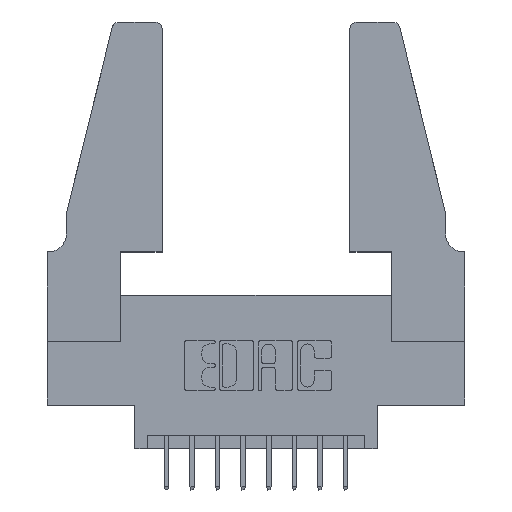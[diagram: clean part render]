
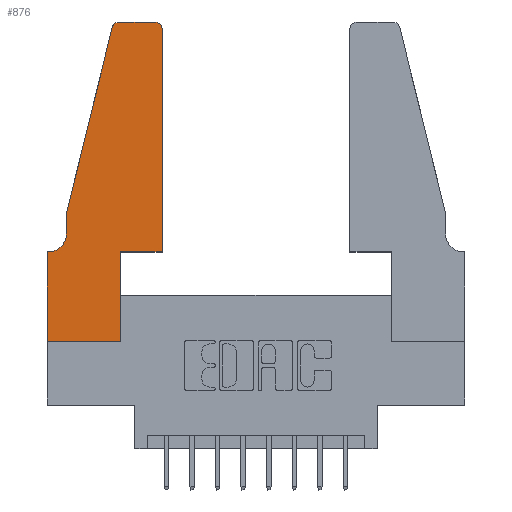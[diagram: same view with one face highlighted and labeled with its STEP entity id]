
A CAD part, top view. The second image highlights one B-rep face of the part: STEP entity #876.
In plain terms, the highlighted planar face has unit normal (0, 0, 1).
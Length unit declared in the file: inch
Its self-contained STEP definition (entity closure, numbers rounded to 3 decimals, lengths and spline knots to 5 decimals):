
#2 = EDGE_CURVE ( 'NONE', #5639, #6989, #9946, .T. ) ;
#331 = VERTEX_POINT ( 'NONE', #1885 ) ;
#429 = EDGE_CURVE ( 'NONE', #331, #4525, #10278, .T. ) ;
#537 = LINE ( 'NONE', #7313, #11053 ) ;
#578 = EDGE_CURVE ( 'NONE', #9862, #8758, #537, .T. ) ;
#680 = ORIENTED_EDGE ( 'NONE', *, *, #429, .T. ) ;
#696 = EDGE_CURVE ( 'NONE', #8758, #331, #12492, .T. ) ;
#757 = DIRECTION ( 'NONE',  ( 0., 1., 0. ) ) ;
#809 = VERTEX_POINT ( 'NONE', #13026 ) ;
#876 = ADVANCED_FACE ( 'NONE', ( #4827 ), #5006, .T. ) ;
#889 = CARTESIAN_POINT ( 'NONE',  ( 0., 0.35, 0.37 ) ) ;
#1090 = DIRECTION ( 'NONE',  ( 1., 0., 0. ) ) ;
#1103 = DIRECTION ( 'NONE',  ( 0., 0., 1. ) ) ;
#1106 = ORIENTED_EDGE ( 'NONE', *, *, #2, .T. ) ;
#1365 = DIRECTION ( 'NONE',  ( 1., 0., 0. ) ) ;
#1399 = VECTOR ( 'NONE', #11381, 39.37008 ) ;
#1441 = VECTOR ( 'NONE', #6751, 39.37008 ) ;
#1780 = CARTESIAN_POINT ( 'NONE',  ( 0.4505, 1.22, 0.37 ) ) ;
#1885 = CARTESIAN_POINT ( 'NONE',  ( 0.0755, 0.42, 0.37 ) ) ;
#1956 = VERTEX_POINT ( 'NONE', #6237 ) ;
#1975 = AXIS2_PLACEMENT_3D ( 'NONE', #5099, #12222, #6137 ) ;
#2273 = EDGE_CURVE ( 'NONE', #11721, #809, #9568, .T. ) ;
#2358 = VECTOR ( 'NONE', #8477, 39.37008 ) ;
#2512 = DIRECTION ( 'NONE',  ( -1., 0., 0. ) ) ;
#3281 = DIRECTION ( 'NONE',  ( -0.239, -0.971, 0. ) ) ;
#3434 = VECTOR ( 'NONE', #1090, 39.37008 ) ;
#3533 = DIRECTION ( 'NONE',  ( 0., 0., 1. ) ) ;
#3571 = ORIENTED_EDGE ( 'NONE', *, *, #10720, .T. ) ;
#3953 = VECTOR ( 'NONE', #2512, 39.37008 ) ;
#4116 = CARTESIAN_POINT ( 'NONE',  ( 0.2865, 0.35, 0.37 ) ) ;
#4489 = CARTESIAN_POINT ( 'NONE',  ( 0., 0.35, 0.37 ) ) ;
#4525 = VERTEX_POINT ( 'NONE', #7285 ) ;
#4594 = VECTOR ( 'NONE', #1365, 39.37008 ) ;
#4827 = FACE_OUTER_BOUND ( 'NONE', #7595, .T. ) ;
#5006 = PLANE ( 'NONE',  #10606 ) ;
#5099 = CARTESIAN_POINT ( 'NONE',  ( 0.0055, 0.42, 0.37 ) ) ;
#5154 = CARTESIAN_POINT ( 'NONE',  ( 0.2865, 0.35, 0.37 ) ) ;
#5297 = ORIENTED_EDGE ( 'NONE', *, *, #2273, .T. ) ;
#5469 = CARTESIAN_POINT ( 'NONE',  ( 0., 0., 0.37 ) ) ;
#5639 = VERTEX_POINT ( 'NONE', #11749 ) ;
#5729 = CARTESIAN_POINT ( 'NONE',  ( 0., 0., 0.37 ) ) ;
#6007 = EDGE_CURVE ( 'NONE', #1956, #13162, #9523, .T. ) ;
#6020 = DIRECTION ( 'NONE',  ( 1., 0., 0. ) ) ;
#6137 = DIRECTION ( 'NONE',  ( -1., 0., 0. ) ) ;
#6199 = ORIENTED_EDGE ( 'NONE', *, *, #696, .T. ) ;
#6237 = CARTESIAN_POINT ( 'NONE',  ( 0.4505, 0.35, 0.37 ) ) ;
#6663 = LINE ( 'NONE', #9638, #3953 ) ;
#6751 = DIRECTION ( 'NONE',  ( 0., -1., 0. ) ) ;
#6989 = VERTEX_POINT ( 'NONE', #5154 ) ;
#7147 = EDGE_CURVE ( 'NONE', #809, #5639, #12729, .T. ) ;
#7213 = CARTESIAN_POINT ( 'NONE',  ( 0.4205, 1.22, 0.37 ) ) ;
#7243 = EDGE_CURVE ( 'NONE', #4525, #11721, #6663, .T. ) ;
#7249 = VECTOR ( 'NONE', #757, 39.37008 ) ;
#7285 = CARTESIAN_POINT ( 'NONE',  ( 0.0055, 0.35, 0.37 ) ) ;
#7313 = CARTESIAN_POINT ( 'NONE',  ( 0.0755, 0.5, 0.37 ) ) ;
#7450 = CARTESIAN_POINT ( 'NONE',  ( 0.2605, 1.25, 0.37 ) ) ;
#7595 = EDGE_LOOP ( 'NONE', ( #11321, #11504, #7727, #6199, #680, #12653, #5297, #10814, #1106, #3571, #12916, #8755 ) ) ;
#7673 = CARTESIAN_POINT ( 'NONE',  ( 0.284, 1.25, 0.37 ) ) ;
#7707 = CIRCLE ( 'NONE', #8654, 0.03 ) ;
#7727 = ORIENTED_EDGE ( 'NONE', *, *, #578, .T. ) ;
#7777 = EDGE_CURVE ( 'NONE', #9281, #12466, #10493, .T. ) ;
#8235 = CARTESIAN_POINT ( 'NONE',  ( 0.4505, 0.35, 0.37 ) ) ;
#8246 = DIRECTION ( 'NONE',  ( 1., 0., 0. ) ) ;
#8477 = DIRECTION ( 'NONE',  ( -1., 0., 0. ) ) ;
#8654 = AXIS2_PLACEMENT_3D ( 'NONE', #7213, #1103, #8246 ) ;
#8755 = ORIENTED_EDGE ( 'NONE', *, *, #12712, .T. ) ;
#8758 = VERTEX_POINT ( 'NONE', #11666 ) ;
#8842 = LINE ( 'NONE', #8235, #3434 ) ;
#9281 = VERTEX_POINT ( 'NONE', #9360 ) ;
#9360 = CARTESIAN_POINT ( 'NONE',  ( 0.4205, 1.25, 0.37 ) ) ;
#9523 = LINE ( 'NONE', #11334, #1399 ) ;
#9568 = LINE ( 'NONE', #5729, #1441 ) ;
#9591 = DIRECTION ( 'NONE',  ( 0., -1., 0. ) ) ;
#9627 = CARTESIAN_POINT ( 'NONE',  ( 0.284, 1.22, 0.37 ) ) ;
#9638 = CARTESIAN_POINT ( 'NONE',  ( 0.0755, 0.35, 0.37 ) ) ;
#9749 = AXIS2_PLACEMENT_3D ( 'NONE', #9627, #3533, #10654 ) ;
#9862 = VERTEX_POINT ( 'NONE', #12033 ) ;
#9946 = LINE ( 'NONE', #4116, #7249 ) ;
#10278 = CIRCLE ( 'NONE', #1975, 0.07 ) ;
#10493 = LINE ( 'NONE', #7450, #2358 ) ;
#10606 = AXIS2_PLACEMENT_3D ( 'NONE', #889, #12122, #6020 ) ;
#10627 = CARTESIAN_POINT ( 'NONE',  ( 0.0755, 0.5, 0.37 ) ) ;
#10654 = DIRECTION ( 'NONE',  ( 1., 0., 0. ) ) ;
#10720 = EDGE_CURVE ( 'NONE', #6989, #1956, #8842, .T. ) ;
#10814 = ORIENTED_EDGE ( 'NONE', *, *, #7147, .T. ) ;
#11053 = VECTOR ( 'NONE', #3281, 39.37008 ) ;
#11321 = ORIENTED_EDGE ( 'NONE', *, *, #7777, .T. ) ;
#11334 = CARTESIAN_POINT ( 'NONE',  ( 0.4505, 0.35, 0.37 ) ) ;
#11364 = CIRCLE ( 'NONE', #9749, 0.03 ) ;
#11381 = DIRECTION ( 'NONE',  ( 0., 1., 0. ) ) ;
#11504 = ORIENTED_EDGE ( 'NONE', *, *, #13045, .T. ) ;
#11666 = CARTESIAN_POINT ( 'NONE',  ( 0.0755, 0.5, 0.37 ) ) ;
#11721 = VERTEX_POINT ( 'NONE', #4489 ) ;
#11749 = CARTESIAN_POINT ( 'NONE',  ( 0.2865, 0., 0.37 ) ) ;
#12033 = CARTESIAN_POINT ( 'NONE',  ( 0.25487, 1.22718, 0.37 ) ) ;
#12122 = DIRECTION ( 'NONE',  ( 0., 0., 1. ) ) ;
#12164 = VECTOR ( 'NONE', #9591, 39.37008 ) ;
#12222 = DIRECTION ( 'NONE',  ( 0., 0., -1. ) ) ;
#12466 = VERTEX_POINT ( 'NONE', #7673 ) ;
#12492 = LINE ( 'NONE', #10627, #12164 ) ;
#12653 = ORIENTED_EDGE ( 'NONE', *, *, #7243, .T. ) ;
#12712 = EDGE_CURVE ( 'NONE', #13162, #9281, #7707, .T. ) ;
#12729 = LINE ( 'NONE', #5469, #4594 ) ;
#12916 = ORIENTED_EDGE ( 'NONE', *, *, #6007, .T. ) ;
#13026 = CARTESIAN_POINT ( 'NONE',  ( 0., 0., 0.37 ) ) ;
#13045 = EDGE_CURVE ( 'NONE', #12466, #9862, #11364, .T. ) ;
#13162 = VERTEX_POINT ( 'NONE', #1780 ) ;
